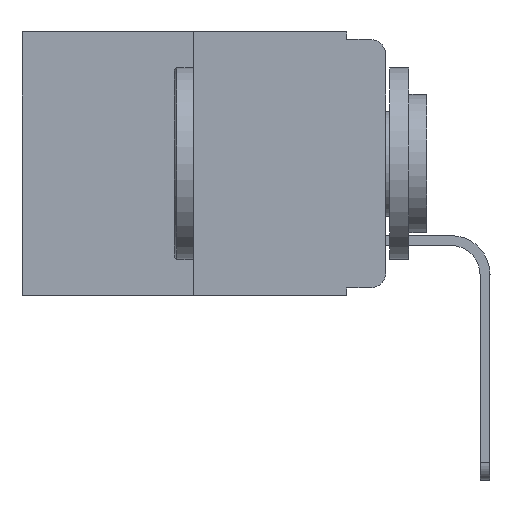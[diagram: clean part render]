
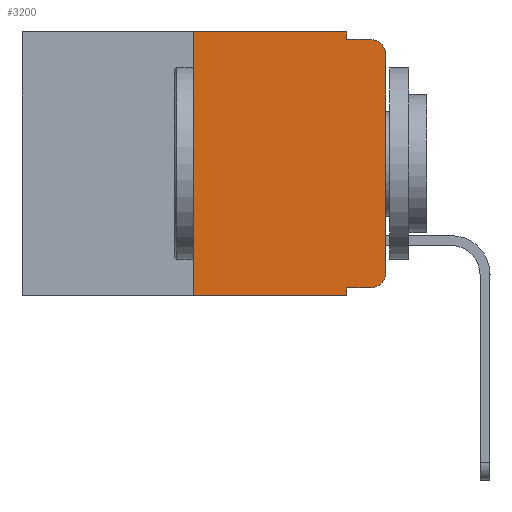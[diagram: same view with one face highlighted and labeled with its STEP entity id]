
A CAD part, left-side view. The second image highlights one B-rep face of the part: STEP entity #3200.
In plain terms, the highlighted planar face has unit normal (-1, 0, 0).
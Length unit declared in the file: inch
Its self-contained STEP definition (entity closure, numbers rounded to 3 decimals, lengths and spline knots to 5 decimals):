
#16 = CARTESIAN_POINT ( 'NONE',  ( 0., 0.02, -0.313 ) ) ;
#63 = DIRECTION ( 'NONE',  ( -1., 0., 0. ) ) ;
#359 = ORIENTED_EDGE ( 'NONE', *, *, #2283, .T. ) ;
#378 = CARTESIAN_POINT ( 'NONE',  ( 0., 0., 0. ) ) ;
#985 = VECTOR ( 'NONE', #8302, 39.37008 ) ;
#1120 = CARTESIAN_POINT ( 'NONE',  ( 0., 0., -0.313 ) ) ;
#1358 = ORIENTED_EDGE ( 'NONE', *, *, #12146, .T. ) ;
#1431 = CARTESIAN_POINT ( 'NONE',  ( 0., 0., -0.03 ) ) ;
#1649 = VERTEX_POINT ( 'NONE', #8517 ) ;
#1743 = VERTEX_POINT ( 'NONE', #11101 ) ;
#1914 = ORIENTED_EDGE ( 'NONE', *, *, #12657, .F. ) ;
#2283 = EDGE_CURVE ( 'NONE', #1743, #10126, #9108, .T. ) ;
#2525 = DIRECTION ( 'NONE',  ( 0., 0., -1. ) ) ;
#2658 = DIRECTION ( 'NONE',  ( 0., 0., -1. ) ) ;
#2670 = ORIENTED_EDGE ( 'NONE', *, *, #6247, .T. ) ;
#3177 = VERTEX_POINT ( 'NONE', #1431 ) ;
#3194 = AXIS2_PLACEMENT_3D ( 'NONE', #10615, #5581, #10482 ) ;
#3200 = ADVANCED_FACE ( 'NONE', ( #8768 ), #11599, .F. ) ;
#3238 = CARTESIAN_POINT ( 'NONE',  ( 0., 0.051, -0.01 ) ) ;
#3379 = VECTOR ( 'NONE', #4262, 39.37008 ) ;
#3742 = VERTEX_POINT ( 'NONE', #5431 ) ;
#3889 = VECTOR ( 'NONE', #2525, 39.37008 ) ;
#4027 = CARTESIAN_POINT ( 'NONE',  ( 0., 0.051, -0.333 ) ) ;
#4171 = CARTESIAN_POINT ( 'NONE',  ( 0., 0.473, -0.343 ) ) ;
#4230 = CARTESIAN_POINT ( 'NONE',  ( 0., 0.02, -0.01 ) ) ;
#4256 = ORIENTED_EDGE ( 'NONE', *, *, #12446, .F. ) ;
#4262 = DIRECTION ( 'NONE',  ( 0., 0., 1. ) ) ;
#4276 = VECTOR ( 'NONE', #7164, 39.37008 ) ;
#4302 = VECTOR ( 'NONE', #7363, 39.37008 ) ;
#4693 = LINE ( 'NONE', #9457, #3889 ) ;
#4829 = CARTESIAN_POINT ( 'NONE',  ( 0., 0.051, -0.333 ) ) ;
#5266 = AXIS2_PLACEMENT_3D ( 'NONE', #12635, #7654, #2658 ) ;
#5301 = VERTEX_POINT ( 'NONE', #9314 ) ;
#5309 = CARTESIAN_POINT ( 'NONE',  ( 0., 0.473, 0. ) ) ;
#5333 = DIRECTION ( 'NONE',  ( 0., -1., 0. ) ) ;
#5431 = CARTESIAN_POINT ( 'NONE',  ( 0., 0.051, -0.01 ) ) ;
#5552 = ORIENTED_EDGE ( 'NONE', *, *, #12500, .T. ) ;
#5581 = DIRECTION ( 'NONE',  ( -1., 0., 0. ) ) ;
#5933 = ORIENTED_EDGE ( 'NONE', *, *, #9295, .T. ) ;
#6092 = VERTEX_POINT ( 'NONE', #4829 ) ;
#6213 = CARTESIAN_POINT ( 'NONE',  ( 0., 0.051, 0. ) ) ;
#6247 = EDGE_CURVE ( 'NONE', #6092, #1649, #9936, .T. ) ;
#6938 = AXIS2_PLACEMENT_3D ( 'NONE', #16, #63, #12116 ) ;
#7164 = DIRECTION ( 'NONE',  ( 0., -1., 0. ) ) ;
#7363 = DIRECTION ( 'NONE',  ( 0., 0., 1. ) ) ;
#7391 = LINE ( 'NONE', #5309, #985 ) ;
#7654 = DIRECTION ( 'NONE',  ( 1., 0., 0. ) ) ;
#7834 = CARTESIAN_POINT ( 'NONE',  ( 0., 0.051, 0. ) ) ;
#7902 = CARTESIAN_POINT ( 'NONE',  ( 0., 0.051, -0.343 ) ) ;
#8020 = VECTOR ( 'NONE', #8117, 39.37008 ) ;
#8047 = EDGE_CURVE ( 'NONE', #5301, #12701, #7391, .T. ) ;
#8117 = DIRECTION ( 'NONE',  ( 0., -1., 0. ) ) ;
#8302 = DIRECTION ( 'NONE',  ( 0., -1., 0. ) ) ;
#8417 = CIRCLE ( 'NONE', #3194, 0.02 ) ;
#8517 = CARTESIAN_POINT ( 'NONE',  ( 0., 0.02, -0.333 ) ) ;
#8768 = FACE_OUTER_BOUND ( 'NONE', #11057, .T. ) ;
#8917 = ORIENTED_EDGE ( 'NONE', *, *, #8047, .F. ) ;
#8943 = CIRCLE ( 'NONE', #6938, 0.02 ) ;
#9108 = LINE ( 'NONE', #4171, #8020 ) ;
#9148 = VERTEX_POINT ( 'NONE', #1120 ) ;
#9195 = EDGE_CURVE ( 'NONE', #12701, #3742, #4693, .T. ) ;
#9216 = CARTESIAN_POINT ( 'NONE',  ( 0., 0.25, 0. ) ) ;
#9295 = EDGE_CURVE ( 'NONE', #3177, #12609, #8417, .T. ) ;
#9314 = CARTESIAN_POINT ( 'NONE',  ( 0., 0.25, 0. ) ) ;
#9457 = CARTESIAN_POINT ( 'NONE',  ( 0., 0.051, 0. ) ) ;
#9844 = DIRECTION ( 'NONE',  ( 0., 0., -1. ) ) ;
#9927 = LINE ( 'NONE', #9216, #3379 ) ;
#9936 = LINE ( 'NONE', #4027, #11206 ) ;
#10126 = VERTEX_POINT ( 'NONE', #7902 ) ;
#10187 = LINE ( 'NONE', #3238, #4276 ) ;
#10482 = DIRECTION ( 'NONE',  ( 0., 0., -1. ) ) ;
#10615 = CARTESIAN_POINT ( 'NONE',  ( 0., 0.02, -0.03 ) ) ;
#11057 = EDGE_LOOP ( 'NONE', ( #1358, #5933, #1914, #12855, #8917, #11207, #359, #4256, #2670, #5552 ) ) ;
#11101 = CARTESIAN_POINT ( 'NONE',  ( 0., 0.25, -0.343 ) ) ;
#11206 = VECTOR ( 'NONE', #5333, 39.37008 ) ;
#11207 = ORIENTED_EDGE ( 'NONE', *, *, #11294, .F. ) ;
#11294 = EDGE_CURVE ( 'NONE', #1743, #5301, #9927, .T. ) ;
#11471 = LINE ( 'NONE', #7834, #11613 ) ;
#11599 = PLANE ( 'NONE',  #5266 ) ;
#11613 = VECTOR ( 'NONE', #9844, 39.37008 ) ;
#11626 = LINE ( 'NONE', #378, #4302 ) ;
#12116 = DIRECTION ( 'NONE',  ( 0., 0., -1. ) ) ;
#12146 = EDGE_CURVE ( 'NONE', #9148, #3177, #11626, .T. ) ;
#12446 = EDGE_CURVE ( 'NONE', #6092, #10126, #11471, .T. ) ;
#12500 = EDGE_CURVE ( 'NONE', #1649, #9148, #8943, .T. ) ;
#12609 = VERTEX_POINT ( 'NONE', #4230 ) ;
#12635 = CARTESIAN_POINT ( 'NONE',  ( 0., 0.473, 0. ) ) ;
#12657 = EDGE_CURVE ( 'NONE', #3742, #12609, #10187, .T. ) ;
#12701 = VERTEX_POINT ( 'NONE', #6213 ) ;
#12855 = ORIENTED_EDGE ( 'NONE', *, *, #9195, .F. ) ;
